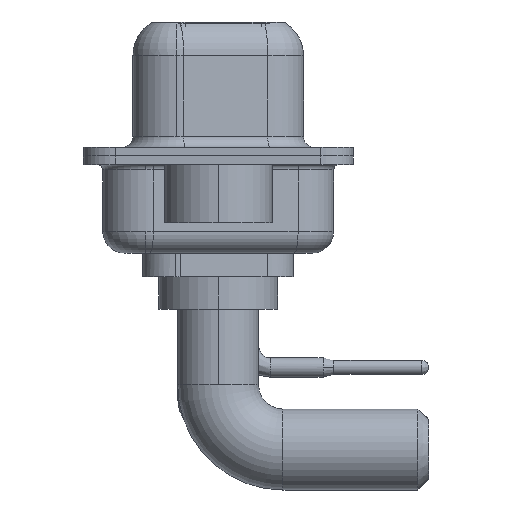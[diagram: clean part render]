
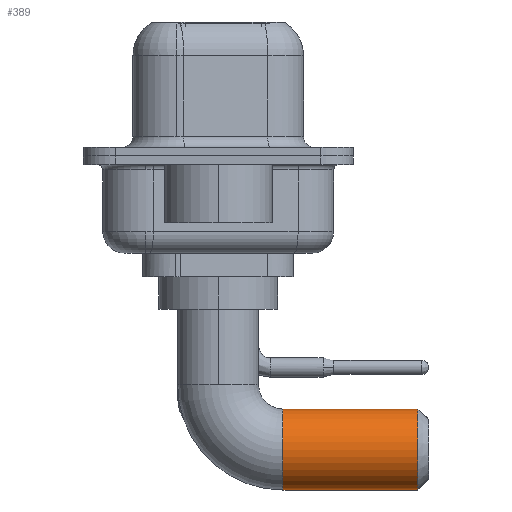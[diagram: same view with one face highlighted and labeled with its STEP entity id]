
A CAD part, left-side view. The second image highlights one B-rep face of the part: STEP entity #389.
In plain terms, the highlighted cylindrical face has radius 1.875 mm (diameter 3.75 mm), a partial arc.
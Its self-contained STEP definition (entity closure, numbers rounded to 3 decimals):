
#273 = CYLINDRICAL_SURFACE ( 'NONE', #10651, 1.875 ) ;
#389 = ADVANCED_FACE ( 'NONE', ( #9116 ), #273, .T. ) ;
#954 = CARTESIAN_POINT ( 'NONE',  ( 0., -3., -4.625 ) ) ;
#1337 = EDGE_CURVE ( 'NONE', #11306, #6595, #1338, .T. ) ;
#1338 = CIRCLE ( 'NONE', #14560, 1.875 ) ;
#1510 = CARTESIAN_POINT ( 'NONE',  ( 0., -3., -4.625 ) ) ;
#3317 = EDGE_CURVE ( 'NONE', #16486, #11306, #11290, .T. ) ;
#3352 = DIRECTION ( 'NONE',  ( 0., -1., 0. ) ) ;
#3690 = ORIENTED_EDGE ( 'NONE', *, *, #1337, .T. ) ;
#3795 = CARTESIAN_POINT ( 'NONE',  ( 0., -3., -8.375 ) ) ;
#4487 = DIRECTION ( 'NONE',  ( 0., 0., -1. ) ) ;
#5274 = DIRECTION ( 'NONE',  ( 0., -1., 0. ) ) ;
#5575 = CARTESIAN_POINT ( 'NONE',  ( 0., -9.25, -4.625 ) ) ;
#6186 = CARTESIAN_POINT ( 'NONE',  ( 0., -9.25, -6.5 ) ) ;
#6312 = VECTOR ( 'NONE', #5274, 1000. ) ;
#6595 = VERTEX_POINT ( 'NONE', #5575 ) ;
#6909 = LINE ( 'NONE', #954, #6312 ) ;
#7189 = EDGE_LOOP ( 'NONE', ( #18146, #14237, #13472, #3690 ) ) ;
#7915 = AXIS2_PLACEMENT_3D ( 'NONE', #12375, #13825, #13913 ) ;
#8587 = EDGE_CURVE ( 'NONE', #12722, #16486, #10065, .T. ) ;
#9116 = FACE_OUTER_BOUND ( 'NONE', #7189, .T. ) ;
#10065 = CIRCLE ( 'NONE', #7915, 1.875 ) ;
#10651 = AXIS2_PLACEMENT_3D ( 'NONE', #14903, #3352, #4487 ) ;
#10684 = CARTESIAN_POINT ( 'NONE',  ( 0., -3., -8.375 ) ) ;
#11290 = LINE ( 'NONE', #3795, #16942 ) ;
#11306 = VERTEX_POINT ( 'NONE', #11459 ) ;
#11459 = CARTESIAN_POINT ( 'NONE',  ( 0., -9.25, -8.375 ) ) ;
#12375 = CARTESIAN_POINT ( 'NONE',  ( 0., -3., -6.5 ) ) ;
#12722 = VERTEX_POINT ( 'NONE', #1510 ) ;
#13472 = ORIENTED_EDGE ( 'NONE', *, *, #3317, .T. ) ;
#13825 = DIRECTION ( 'NONE',  ( 0., -1., 0. ) ) ;
#13913 = DIRECTION ( 'NONE',  ( -1., 0., 0. ) ) ;
#14237 = ORIENTED_EDGE ( 'NONE', *, *, #8587, .T. ) ;
#14560 = AXIS2_PLACEMENT_3D ( 'NONE', #6186, #16208, #17557 ) ;
#14903 = CARTESIAN_POINT ( 'NONE',  ( 0., -3., -6.5 ) ) ;
#15676 = EDGE_CURVE ( 'NONE', #12722, #6595, #6909, .T. ) ;
#16208 = DIRECTION ( 'NONE',  ( 0., 1., 0. ) ) ;
#16486 = VERTEX_POINT ( 'NONE', #10684 ) ;
#16942 = VECTOR ( 'NONE', #17184, 1000. ) ;
#17184 = DIRECTION ( 'NONE',  ( 0., -1., 0. ) ) ;
#17557 = DIRECTION ( 'NONE',  ( 0., 0., -1. ) ) ;
#18146 = ORIENTED_EDGE ( 'NONE', *, *, #15676, .F. ) ;
